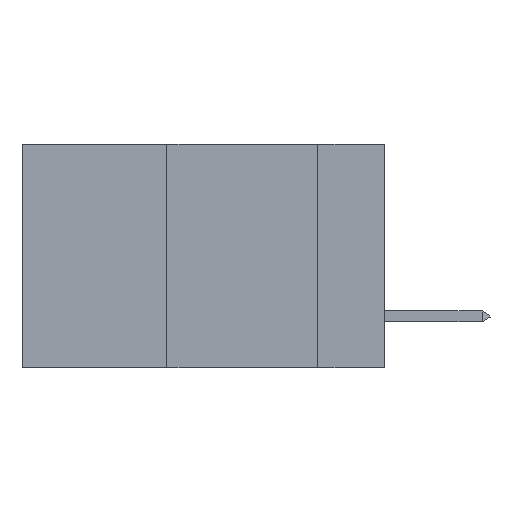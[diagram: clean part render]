
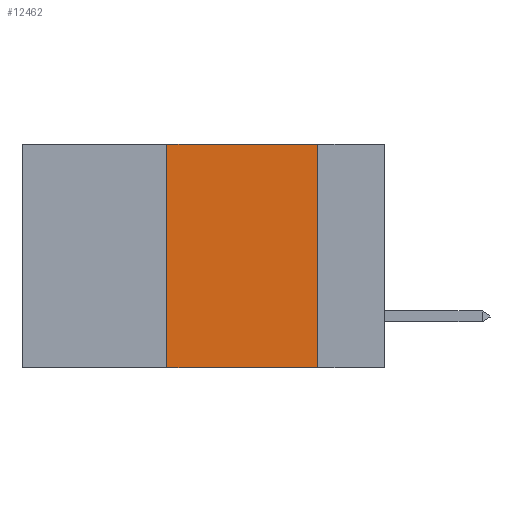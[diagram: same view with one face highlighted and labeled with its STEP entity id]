
A CAD part, left-side view. The second image highlights one B-rep face of the part: STEP entity #12462.
In plain terms, the highlighted planar face has unit normal (-1, 0, 0).
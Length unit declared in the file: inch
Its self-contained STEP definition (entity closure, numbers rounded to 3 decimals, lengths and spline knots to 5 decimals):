
#3118 = ORIENTED_EDGE ( 'NONE', *, *, #20271, .F. ) ;
#7315 = CARTESIAN_POINT ( 'NONE',  ( 0., 0.11, 0. ) ) ;
#7852 = VERTEX_POINT ( 'NONE', #12143 ) ;
#10564 = CARTESIAN_POINT ( 'NONE',  ( 0., 0.11, 0. ) ) ;
#11387 = DIRECTION ( 'NONE',  ( 0., -1., 0. ) ) ;
#11480 = ORIENTED_EDGE ( 'NONE', *, *, #18092, .T. ) ;
#12143 = CARTESIAN_POINT ( 'NONE',  ( 0., 0.36, -0.37 ) ) ;
#12462 = ADVANCED_FACE ( 'NONE', ( #23080 ), #13955, .F. ) ;
#13414 = LINE ( 'NONE', #10564, #27852 ) ;
#13513 = CARTESIAN_POINT ( 'NONE',  ( 0., 0.11, -0.37 ) ) ;
#13789 = LINE ( 'NONE', #38937, #30665 ) ;
#13955 = PLANE ( 'NONE',  #23687 ) ;
#17099 = CARTESIAN_POINT ( 'NONE',  ( 0., 0.6, 0. ) ) ;
#18092 = EDGE_CURVE ( 'NONE', #7852, #34864, #27876, .T. ) ;
#19272 = ORIENTED_EDGE ( 'NONE', *, *, #32148, .F. ) ;
#20271 = EDGE_CURVE ( 'NONE', #30188, #34864, #13414, .T. ) ;
#20550 = CARTESIAN_POINT ( 'NONE',  ( 0., 0.36, 0. ) ) ;
#20977 = CARTESIAN_POINT ( 'NONE',  ( 0., 0.6, -0.37 ) ) ;
#21138 = VERTEX_POINT ( 'NONE', #26369 ) ;
#23080 = FACE_OUTER_BOUND ( 'NONE', #27896, .T. ) ;
#23498 = DIRECTION ( 'NONE',  ( 0., 0., -1. ) ) ;
#23587 = DIRECTION ( 'NONE',  ( 0., 0., 1. ) ) ;
#23687 = AXIS2_PLACEMENT_3D ( 'NONE', #17099, #29172, #23498 ) ;
#24310 = LINE ( 'NONE', #20550, #28624 ) ;
#25484 = DIRECTION ( 'NONE',  ( 0., 0., -1. ) ) ;
#25947 = EDGE_CURVE ( 'NONE', #21138, #30188, #13789, .T. ) ;
#26369 = CARTESIAN_POINT ( 'NONE',  ( 0., 0.36, 0. ) ) ;
#27852 = VECTOR ( 'NONE', #25484, 39.37008 ) ;
#27876 = LINE ( 'NONE', #20977, #37036 ) ;
#27896 = EDGE_LOOP ( 'NONE', ( #3118, #33696, #19272, #11480 ) ) ;
#28624 = VECTOR ( 'NONE', #23587, 39.37008 ) ;
#29172 = DIRECTION ( 'NONE',  ( 1., 0., 0. ) ) ;
#30188 = VERTEX_POINT ( 'NONE', #7315 ) ;
#30665 = VECTOR ( 'NONE', #11387, 39.37008 ) ;
#32148 = EDGE_CURVE ( 'NONE', #7852, #21138, #24310, .T. ) ;
#33696 = ORIENTED_EDGE ( 'NONE', *, *, #25947, .F. ) ;
#34864 = VERTEX_POINT ( 'NONE', #13513 ) ;
#37036 = VECTOR ( 'NONE', #39376, 39.37008 ) ;
#38937 = CARTESIAN_POINT ( 'NONE',  ( 0., 0.6, 0. ) ) ;
#39376 = DIRECTION ( 'NONE',  ( 0., -1., 0. ) ) ;
